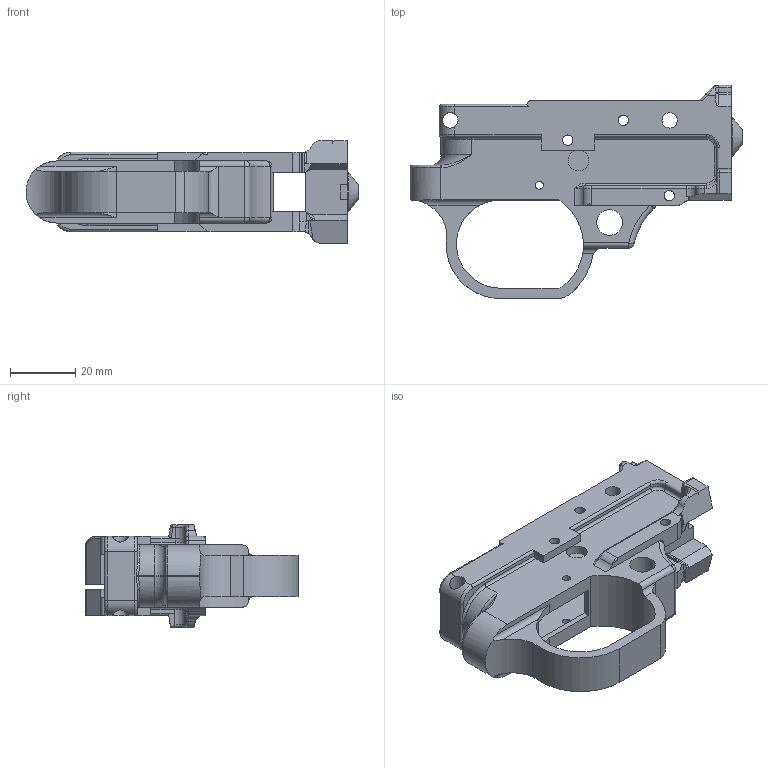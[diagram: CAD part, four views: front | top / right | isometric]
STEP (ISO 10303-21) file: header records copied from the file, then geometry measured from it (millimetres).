
FILE_DESCRIPTION((''),'2;1');
FILE_NAME('Trigger Housing.stp','2011-10-06T13:13:24',('Bob'),(''),'Autodesk Inventor 2011','Autodesk Inventor 2011','');
FILE_SCHEMA(('AUTOMOTIVE_DESIGN { 1 0 10303 214 1 1 1 1 }'));
Length unit declared in the file: inch
Products named in the file (1): Trigger Housing
Bounding box: 102.03 x 65.49 x 31.6 mm (x, y, z)
Volume: 39981.1 mm3; surface area: 20858.7 mm2
Topology: 1 solids, 1 shells, 246 faces, 687 edges, 426 vertices
Faces by surface type: cylinder 100, plane 91, torus 29, bspline 19, sphere 6, cone 1
Full cylindrical faces by diameter (mm): 2.438 x2, 3.175 x6, 3.759 x1, 4.763 x3, 6.35 x1, 7.938 x1, 12.192 x1
Entity records: 8547 total; most frequent: CARTESIAN_POINT 2305, ORIENTED_EDGE 1312, DIRECTION 1286, EDGE_CURVE 656, AXIS2_PLACEMENT_3D 475, VERTEX_POINT 419, VECTOR 336, LINE 336
